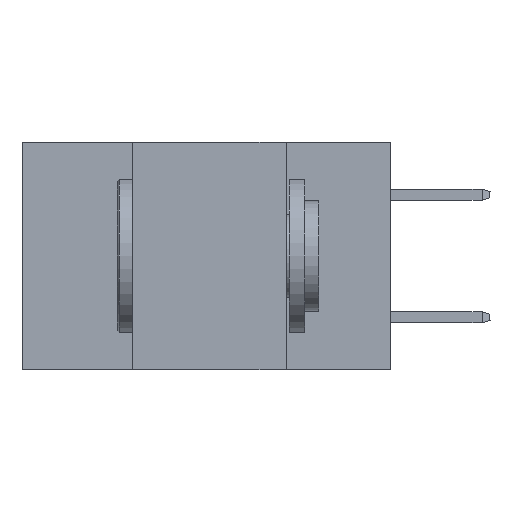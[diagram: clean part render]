
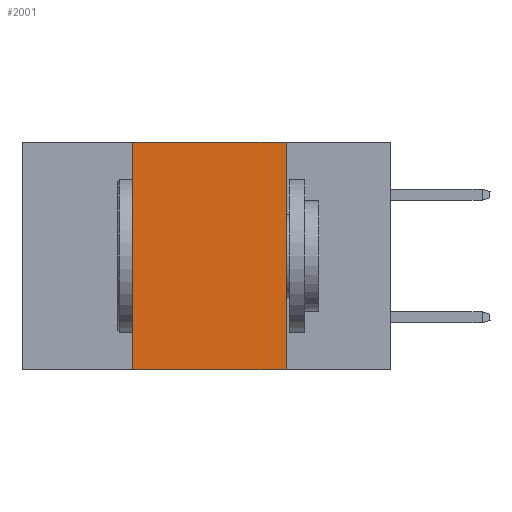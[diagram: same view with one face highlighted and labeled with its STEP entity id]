
A CAD part, left-side view. The second image highlights one B-rep face of the part: STEP entity #2001.
In plain terms, the highlighted planar face has unit normal (-1, 0, 0).
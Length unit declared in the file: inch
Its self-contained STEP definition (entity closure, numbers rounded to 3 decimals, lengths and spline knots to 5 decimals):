
#807 = DIRECTION ( 'NONE',  ( 0., 0., -1. ) ) ;
#1869 = VECTOR ( 'NONE', #20144, 39.37008 ) ;
#2001 = ADVANCED_FACE ( 'NONE', ( #20946 ), #5594, .F. ) ;
#2717 = ORIENTED_EDGE ( 'NONE', *, *, #31257, .T. ) ;
#4099 = VECTOR ( 'NONE', #807, 39.37008 ) ;
#5594 = PLANE ( 'NONE',  #35117 ) ;
#7158 = CARTESIAN_POINT ( 'NONE',  ( 0., 0.17, 0. ) ) ;
#8817 = CARTESIAN_POINT ( 'NONE',  ( 0., 0.6, 0. ) ) ;
#9815 = EDGE_CURVE ( 'NONE', #34881, #38374, #25899, .T. ) ;
#10891 = VERTEX_POINT ( 'NONE', #13035 ) ;
#11848 = CARTESIAN_POINT ( 'NONE',  ( 0., 0.6, -0.37 ) ) ;
#12004 = DIRECTION ( 'NONE',  ( 0., 0., -1. ) ) ;
#12343 = ORIENTED_EDGE ( 'NONE', *, *, #9815, .F. ) ;
#12776 = ORIENTED_EDGE ( 'NONE', *, *, #14551, .F. ) ;
#12948 = CARTESIAN_POINT ( 'NONE',  ( 0., 0.6, 0. ) ) ;
#13035 = CARTESIAN_POINT ( 'NONE',  ( 0., 0.17, 0. ) ) ;
#14551 = EDGE_CURVE ( 'NONE', #10891, #17527, #26088, .T. ) ;
#14698 = LINE ( 'NONE', #12948, #20983 ) ;
#17527 = VERTEX_POINT ( 'NONE', #25277 ) ;
#17615 = LINE ( 'NONE', #11848, #32007 ) ;
#18766 = EDGE_LOOP ( 'NONE', ( #12776, #25855, #12343, #2717 ) ) ;
#20144 = DIRECTION ( 'NONE',  ( 0., 0., 1. ) ) ;
#20946 = FACE_OUTER_BOUND ( 'NONE', #18766, .T. ) ;
#20983 = VECTOR ( 'NONE', #31368, 39.37008 ) ;
#22469 = EDGE_CURVE ( 'NONE', #38374, #10891, #14698, .T. ) ;
#25277 = CARTESIAN_POINT ( 'NONE',  ( 0., 0.17, -0.37 ) ) ;
#25855 = ORIENTED_EDGE ( 'NONE', *, *, #22469, .F. ) ;
#25899 = LINE ( 'NONE', #38538, #1869 ) ;
#26088 = LINE ( 'NONE', #7158, #4099 ) ;
#26976 = CARTESIAN_POINT ( 'NONE',  ( 0., 0.42, -0.37 ) ) ;
#27240 = DIRECTION ( 'NONE',  ( 0., -1., 0. ) ) ;
#30437 = DIRECTION ( 'NONE',  ( 1., 0., 0. ) ) ;
#31257 = EDGE_CURVE ( 'NONE', #34881, #17527, #17615, .T. ) ;
#31368 = DIRECTION ( 'NONE',  ( 0., -1., 0. ) ) ;
#32007 = VECTOR ( 'NONE', #27240, 39.37008 ) ;
#34881 = VERTEX_POINT ( 'NONE', #26976 ) ;
#35117 = AXIS2_PLACEMENT_3D ( 'NONE', #8817, #30437, #12004 ) ;
#35710 = CARTESIAN_POINT ( 'NONE',  ( 0., 0.42, 0. ) ) ;
#38374 = VERTEX_POINT ( 'NONE', #35710 ) ;
#38538 = CARTESIAN_POINT ( 'NONE',  ( 0., 0.42, 0. ) ) ;
